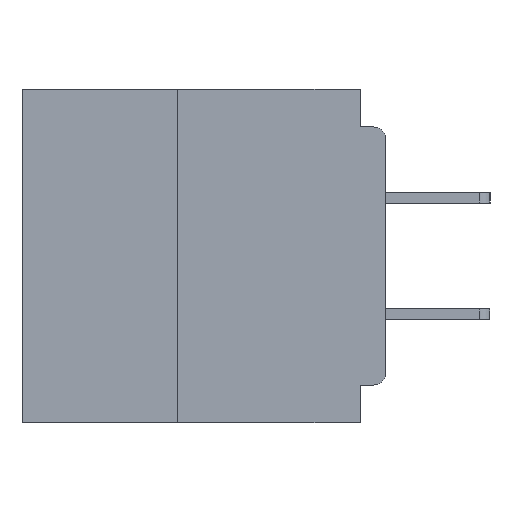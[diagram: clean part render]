
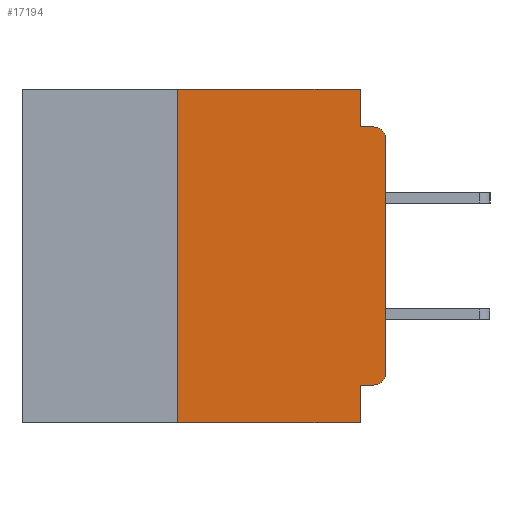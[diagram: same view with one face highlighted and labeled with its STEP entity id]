
A CAD part, left-side view. The second image highlights one B-rep face of the part: STEP entity #17194.
In plain terms, the highlighted planar face has unit normal (-1, 0, 0).
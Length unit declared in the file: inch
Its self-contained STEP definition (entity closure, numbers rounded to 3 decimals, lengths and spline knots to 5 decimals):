
#471 = CARTESIAN_POINT ( 'NONE',  ( 0., 0.015, -0.045 ) ) ;
#1222 = VERTEX_POINT ( 'NONE', #471 ) ;
#3013 = ORIENTED_EDGE ( 'NONE', *, *, #34789, .F. ) ;
#3299 = CARTESIAN_POINT ( 'NONE',  ( 0., 0.015, -0.355 ) ) ;
#3408 = EDGE_CURVE ( 'NONE', #35578, #3581, #22577, .T. ) ;
#3581 = VERTEX_POINT ( 'NONE', #5700 ) ;
#3996 = CARTESIAN_POINT ( 'NONE',  ( 0., 0.25, -0.4 ) ) ;
#4037 = LINE ( 'NONE', #26213, #28012 ) ;
#4041 = CARTESIAN_POINT ( 'NONE',  ( 0., 0.25, 0. ) ) ;
#4400 = LINE ( 'NONE', #3996, #19171 ) ;
#5255 = EDGE_CURVE ( 'NONE', #12670, #19511, #15096, .T. ) ;
#5332 = EDGE_LOOP ( 'NONE', ( #33294, #20660, #19649, #40286, #31568, #17434, #26878, #3013, #30459, #5883 ) ) ;
#5700 = CARTESIAN_POINT ( 'NONE',  ( 0., 0.031, -0.4 ) ) ;
#5782 = CIRCLE ( 'NONE', #34840, 0.015 ) ;
#5883 = ORIENTED_EDGE ( 'NONE', *, *, #27470, .T. ) ;
#6452 = CARTESIAN_POINT ( 'NONE',  ( 0., 0.437, 0. ) ) ;
#7620 = CARTESIAN_POINT ( 'NONE',  ( 0., 0., -0.34 ) ) ;
#7684 = LINE ( 'NONE', #6452, #24347 ) ;
#10060 = DIRECTION ( 'NONE',  ( -1., 0., 0. ) ) ;
#10419 = DIRECTION ( 'NONE',  ( -1., 0., 0. ) ) ;
#10474 = CARTESIAN_POINT ( 'NONE',  ( 0., 0.031, -0.355 ) ) ;
#10825 = DIRECTION ( 'NONE',  ( 0., 0., -1. ) ) ;
#10835 = CARTESIAN_POINT ( 'NONE',  ( 0., 0., -0.06 ) ) ;
#11443 = CARTESIAN_POINT ( 'NONE',  ( 0., 0.031, -0.045 ) ) ;
#12095 = CARTESIAN_POINT ( 'NONE',  ( 0., 0.437, -0.4 ) ) ;
#12670 = VERTEX_POINT ( 'NONE', #7620 ) ;
#12798 = VECTOR ( 'NONE', #22264, 39.37008 ) ;
#15096 = LINE ( 'NONE', #23060, #27722 ) ;
#15774 = EDGE_CURVE ( 'NONE', #27393, #39979, #21117, .T. ) ;
#15807 = VERTEX_POINT ( 'NONE', #25499 ) ;
#16468 = DIRECTION ( 'NONE',  ( 0., -1., 0. ) ) ;
#16972 = CARTESIAN_POINT ( 'NONE',  ( 0., 0.25, -0.4 ) ) ;
#16979 = CARTESIAN_POINT ( 'NONE',  ( 0., 0.437, 0. ) ) ;
#17194 = ADVANCED_FACE ( 'NONE', ( #25342 ), #35342, .F. ) ;
#17214 = DIRECTION ( 'NONE',  ( 0., -1., 0. ) ) ;
#17434 = ORIENTED_EDGE ( 'NONE', *, *, #31333, .F. ) ;
#17646 = AXIS2_PLACEMENT_3D ( 'NONE', #16979, #38583, #20132 ) ;
#19171 = VECTOR ( 'NONE', #19818, 39.37008 ) ;
#19511 = VERTEX_POINT ( 'NONE', #10835 ) ;
#19649 = ORIENTED_EDGE ( 'NONE', *, *, #24892, .F. ) ;
#19818 = DIRECTION ( 'NONE',  ( 0., 0., 1. ) ) ;
#20132 = DIRECTION ( 'NONE',  ( 0., 0., -1. ) ) ;
#20660 = ORIENTED_EDGE ( 'NONE', *, *, #22901, .T. ) ;
#21117 = LINE ( 'NONE', #28337, #12798 ) ;
#22264 = DIRECTION ( 'NONE',  ( 0., 1., 0. ) ) ;
#22577 = LINE ( 'NONE', #12095, #38922 ) ;
#22901 = EDGE_CURVE ( 'NONE', #19511, #1222, #34057, .T. ) ;
#23000 = DIRECTION ( 'NONE',  ( 0., 0., 1. ) ) ;
#23060 = CARTESIAN_POINT ( 'NONE',  ( 0., 0., 0. ) ) ;
#23995 = EDGE_CURVE ( 'NONE', #37235, #15807, #7684, .T. ) ;
#24347 = VECTOR ( 'NONE', #25159, 39.37008 ) ;
#24892 = EDGE_CURVE ( 'NONE', #36337, #1222, #25217, .T. ) ;
#25159 = DIRECTION ( 'NONE',  ( 0., -1., 0. ) ) ;
#25217 = LINE ( 'NONE', #38801, #32432 ) ;
#25342 = FACE_OUTER_BOUND ( 'NONE', #5332, .T. ) ;
#25499 = CARTESIAN_POINT ( 'NONE',  ( 0., 0.031, 0. ) ) ;
#26213 = CARTESIAN_POINT ( 'NONE',  ( 0., 0.031, -0.4 ) ) ;
#26878 = ORIENTED_EDGE ( 'NONE', *, *, #3408, .T. ) ;
#26996 = VECTOR ( 'NONE', #10825, 39.37008 ) ;
#27393 = VERTEX_POINT ( 'NONE', #3299 ) ;
#27470 = EDGE_CURVE ( 'NONE', #27393, #12670, #5782, .T. ) ;
#27722 = VECTOR ( 'NONE', #23000, 39.37008 ) ;
#28012 = VECTOR ( 'NONE', #35486, 39.37008 ) ;
#28337 = CARTESIAN_POINT ( 'NONE',  ( 0., 0., -0.355 ) ) ;
#28739 = CARTESIAN_POINT ( 'NONE',  ( 0., 0.015, -0.34 ) ) ;
#29085 = CARTESIAN_POINT ( 'NONE',  ( 0., 0.015, -0.06 ) ) ;
#29473 = CARTESIAN_POINT ( 'NONE',  ( 0., 0.031, 0. ) ) ;
#30459 = ORIENTED_EDGE ( 'NONE', *, *, #15774, .F. ) ;
#30763 = EDGE_CURVE ( 'NONE', #15807, #36337, #35136, .T. ) ;
#31333 = EDGE_CURVE ( 'NONE', #35578, #37235, #4400, .T. ) ;
#31568 = ORIENTED_EDGE ( 'NONE', *, *, #23995, .F. ) ;
#31805 = DIRECTION ( 'NONE',  ( 0., 0., -1. ) ) ;
#32144 = DIRECTION ( 'NONE',  ( 0., 0., -1. ) ) ;
#32432 = VECTOR ( 'NONE', #17214, 39.37008 ) ;
#33294 = ORIENTED_EDGE ( 'NONE', *, *, #5255, .T. ) ;
#34057 = CIRCLE ( 'NONE', #38193, 0.015 ) ;
#34789 = EDGE_CURVE ( 'NONE', #39979, #3581, #4037, .T. ) ;
#34840 = AXIS2_PLACEMENT_3D ( 'NONE', #28739, #10060, #31805 ) ;
#35136 = LINE ( 'NONE', #29473, #26996 ) ;
#35342 = PLANE ( 'NONE',  #17646 ) ;
#35486 = DIRECTION ( 'NONE',  ( 0., 0., -1. ) ) ;
#35578 = VERTEX_POINT ( 'NONE', #16972 ) ;
#36337 = VERTEX_POINT ( 'NONE', #11443 ) ;
#37235 = VERTEX_POINT ( 'NONE', #4041 ) ;
#38193 = AXIS2_PLACEMENT_3D ( 'NONE', #29085, #10419, #32144 ) ;
#38583 = DIRECTION ( 'NONE',  ( 1., 0., 0. ) ) ;
#38801 = CARTESIAN_POINT ( 'NONE',  ( 0., 0., -0.045 ) ) ;
#38922 = VECTOR ( 'NONE', #16468, 39.37008 ) ;
#39979 = VERTEX_POINT ( 'NONE', #10474 ) ;
#40286 = ORIENTED_EDGE ( 'NONE', *, *, #30763, .F. ) ;
